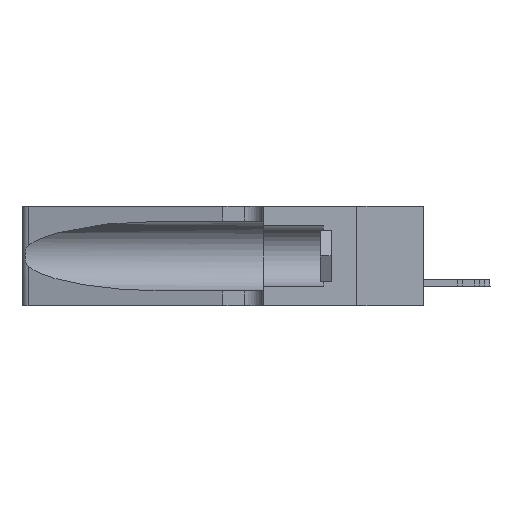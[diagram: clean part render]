
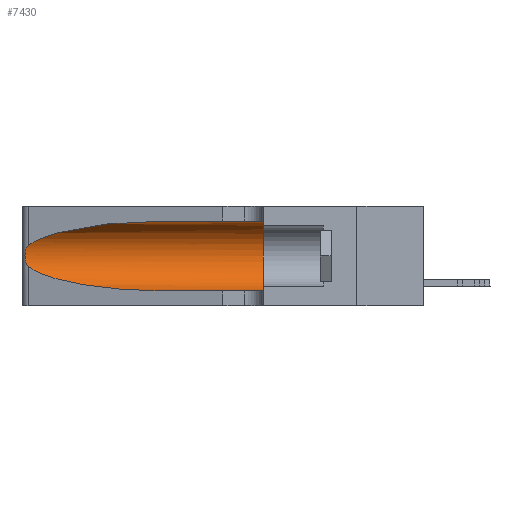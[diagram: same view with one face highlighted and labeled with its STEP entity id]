
A CAD part, left-side view. The second image highlights one B-rep face of the part: STEP entity #7430.
In plain terms, the highlighted cylindrical face has radius 3.308 mm (diameter 6.617 mm), a partial arc.
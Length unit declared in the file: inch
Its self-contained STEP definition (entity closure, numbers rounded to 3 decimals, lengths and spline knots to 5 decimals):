
#533 = CARTESIAN_POINT ( 'NONE',  ( 0.25487, 1.22718, 0.22369 ) ) ;
#1523 = EDGE_CURVE ( 'NONE', #23233, #23009, #32919, .T. ) ;
#2029 = VERTEX_POINT ( 'NONE', #27248 ) ;
#2095 = CARTESIAN_POINT ( 'NONE',  ( 0.1305, 0.72297, 0.05475 ) ) ;
#3757 = VECTOR ( 'NONE', #21628, 39.37008 ) ;
#4032 = CARTESIAN_POINT ( 'NONE',  ( 0.26075, 1.23896, 0.19203 ) ) ;
#4304 = CARTESIAN_POINT ( 'NONE',  ( 0.26017, 1.23833, 0.17102 ) ) ;
#4545 = DIRECTION ( 'NONE',  ( 0., 1., 0. ) ) ;
#4997 = DIRECTION ( 'NONE',  ( 0., 0., -1. ) ) ;
#5892 = DIRECTION ( 'NONE',  ( 0., -1., 0. ) ) ;
#6888 = CARTESIAN_POINT ( 'NONE',  ( 0.2373, 1.15595, 0.08982 ) ) ;
#7267 = CARTESIAN_POINT ( 'NONE',  ( 0.25555, 1.22993, 0.14849 ) ) ;
#7430 = ADVANCED_FACE ( 'NONE', ( #8538 ), #24748, .F. ) ;
#7822 = CARTESIAN_POINT ( 'NONE',  ( 0.26075, 1.23896, 0.178 ) ) ;
#8491 = VERTEX_POINT ( 'NONE', #37053 ) ;
#8538 = FACE_OUTER_BOUND ( 'NONE', #39590, .T. ) ;
#9558 = EDGE_CURVE ( 'NONE', #11954, #8491, #31609, .T. ) ;
#10068 = DIRECTION ( 'NONE',  ( 0., 0., 1. ) ) ;
#10234 = CARTESIAN_POINT ( 'NONE',  ( 0.25487, 1.22718, 0.14631 ) ) ;
#10446 = AXIS2_PLACEMENT_3D ( 'NONE', #27868, #4545, #10068 ) ;
#10509 = CARTESIAN_POINT ( 'NONE',  ( 0.26018, 1.23835, 0.19895 ) ) ;
#10891 = CARTESIAN_POINT ( 'NONE',  ( 0.1305, 0.72297, 0.31525 ) ) ;
#11063 = CARTESIAN_POINT ( 'NONE',  ( 0.25639, 1.23186, 0.15144 ) ) ;
#11249 = CARTESIAN_POINT ( 'NONE',  ( 0.25487, 1.22718, 0.14631 ) ) ;
#11954 = VERTEX_POINT ( 'NONE', #10891 ) ;
#12443 = ORIENTED_EDGE ( 'NONE', *, *, #37880, .F. ) ;
#14041 = CARTESIAN_POINT ( 'NONE',  ( 0.25854, 1.2359, 0.20912 ) ) ;
#14171 = CARTESIAN_POINT ( 'NONE',  ( 0.25487, 1.22718, 0.14631 ) ) ;
#15021 = DIRECTION ( 'NONE',  ( 0., -1., 0. ) ) ;
#16151 =( BOUNDED_CURVE ( )  B_SPLINE_CURVE ( 3, ( #10234, #6888, #26496, #38982 ),
 .UNSPECIFIED., .F., .T. ) 
 B_SPLINE_CURVE_WITH_KNOTS ( ( 4, 4 ),
 ( 3.44316, 4.71239 ),
 .UNSPECIFIED. ) 
 CURVE ( )  GEOMETRIC_REPRESENTATION_ITEM ( )  RATIONAL_B_SPLINE_CURVE ( ( 1., 0.87, 0.87, 1. ) ) 
 REPRESENTATION_ITEM ( '' )  );
#17481 = VECTOR ( 'NONE', #5892, 39.37008 ) ;
#20309 = CARTESIAN_POINT ( 'NONE',  ( 0.18966, 0.96281, 0.31525 ) ) ;
#20823 = CARTESIAN_POINT ( 'NONE',  ( 0.25789, 1.23486, 0.15765 ) ) ;
#21628 = DIRECTION ( 'NONE',  ( 0., -1., 0. ) ) ;
#21812 = CARTESIAN_POINT ( 'NONE',  ( 0.1305, 1.61858, 0.185 ) ) ;
#21954 = CARTESIAN_POINT ( 'NONE',  ( 0.1305, 1.61858, 0.31525 ) ) ;
#23009 = VERTEX_POINT ( 'NONE', #25251 ) ;
#23233 = VERTEX_POINT ( 'NONE', #2095 ) ;
#24748 = CYLINDRICAL_SURFACE ( 'NONE', #26792, 0.13025 ) ;
#24936 =( BOUNDED_CURVE ( )  B_SPLINE_CURVE ( 3, ( #36349, #20309, #26947, #533 ),
 .UNSPECIFIED., .F., .T. ) 
 B_SPLINE_CURVE_WITH_KNOTS ( ( 4, 4 ),
 ( 1.5708, 2.84003 ),
 .UNSPECIFIED. ) 
 CURVE ( )  GEOMETRIC_REPRESENTATION_ITEM ( )  RATIONAL_B_SPLINE_CURVE ( ( 1., 0.87, 0.87, 1. ) ) 
 REPRESENTATION_ITEM ( '' )  );
#25251 = CARTESIAN_POINT ( 'NONE',  ( 0.1305, 0.35, 0.05475 ) ) ;
#26496 = CARTESIAN_POINT ( 'NONE',  ( 0.18966, 0.96281, 0.05475 ) ) ;
#26792 = AXIS2_PLACEMENT_3D ( 'NONE', #21812, #15021, #4997 ) ;
#26947 = CARTESIAN_POINT ( 'NONE',  ( 0.2373, 1.15595, 0.28018 ) ) ;
#26950 = B_SPLINE_CURVE_WITH_KNOTS ( 'NONE', 3,
 ( #27181, #39515, #39784, #40063, #14041, #10509, #4032, #7822, #4304, #30350, #20823, #11063, #7267, #14171 ),
 .UNSPECIFIED., .F., .F.,
 ( 4, 2, 2, 2, 2, 2, 4 ),
 ( 0., 0.00027, 0.00053, 0.00107, 0.0016, 0.00187, 0.00214 ),
 .UNSPECIFIED. ) ;
#27181 = CARTESIAN_POINT ( 'NONE',  ( 0.25487, 1.22718, 0.22369 ) ) ;
#27248 = CARTESIAN_POINT ( 'NONE',  ( 0.25487, 1.22718, 0.22369 ) ) ;
#27868 = CARTESIAN_POINT ( 'NONE',  ( 0.1305, 0.35, 0.185 ) ) ;
#30169 = ORIENTED_EDGE ( 'NONE', *, *, #1523, .T. ) ;
#30350 = CARTESIAN_POINT ( 'NONE',  ( 0.25856, 1.23593, 0.16098 ) ) ;
#31154 = ORIENTED_EDGE ( 'NONE', *, *, #38669, .T. ) ;
#31609 = LINE ( 'NONE', #21954, #17481 ) ;
#32919 = LINE ( 'NONE', #35016, #3757 ) ;
#35016 = CARTESIAN_POINT ( 'NONE',  ( 0.1305, 1.61858, 0.05475 ) ) ;
#36349 = CARTESIAN_POINT ( 'NONE',  ( 0.1305, 0.72297, 0.31525 ) ) ;
#37053 = CARTESIAN_POINT ( 'NONE',  ( 0.1305, 0.35, 0.31525 ) ) ;
#37119 = ORIENTED_EDGE ( 'NONE', *, *, #38785, .T. ) ;
#37880 = EDGE_CURVE ( 'NONE', #8491, #23009, #39031, .T. ) ;
#38669 = EDGE_CURVE ( 'NONE', #41511, #23233, #16151, .T. ) ;
#38785 = EDGE_CURVE ( 'NONE', #2029, #41511, #26950, .T. ) ;
#38982 = CARTESIAN_POINT ( 'NONE',  ( 0.1305, 0.72297, 0.05475 ) ) ;
#39031 = CIRCLE ( 'NONE', #10446, 0.13025 ) ;
#39515 = CARTESIAN_POINT ( 'NONE',  ( 0.25555, 1.22994, 0.2215 ) ) ;
#39590 = EDGE_LOOP ( 'NONE', ( #41275, #37119, #31154, #30169, #12443, #40528 ) ) ;
#39784 = CARTESIAN_POINT ( 'NONE',  ( 0.25639, 1.23184, 0.21858 ) ) ;
#39967 = EDGE_CURVE ( 'NONE', #11954, #2029, #24936, .T. ) ;
#40063 = CARTESIAN_POINT ( 'NONE',  ( 0.25787, 1.23484, 0.2124 ) ) ;
#40528 = ORIENTED_EDGE ( 'NONE', *, *, #9558, .F. ) ;
#41275 = ORIENTED_EDGE ( 'NONE', *, *, #39967, .T. ) ;
#41511 = VERTEX_POINT ( 'NONE', #11249 ) ;
